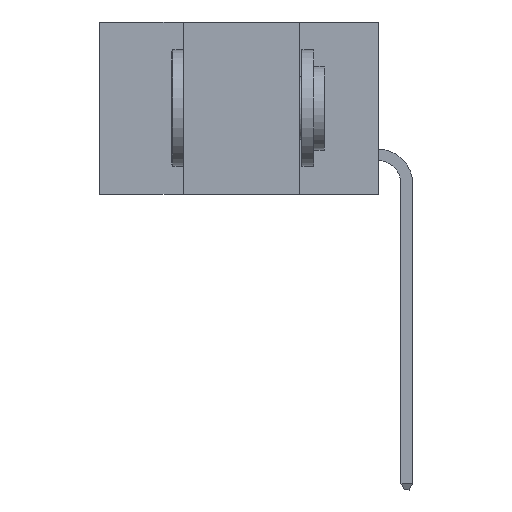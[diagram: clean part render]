
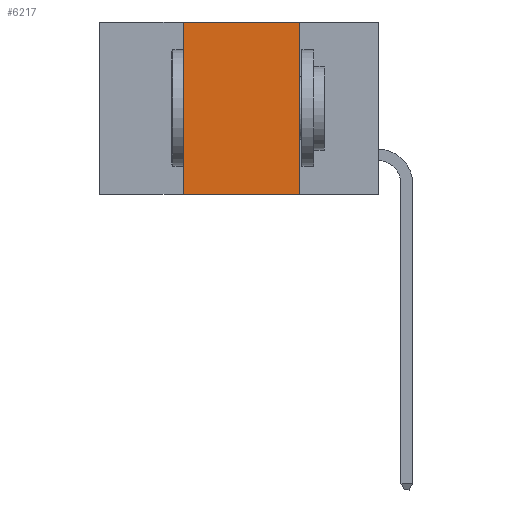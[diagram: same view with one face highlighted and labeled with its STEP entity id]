
A CAD part, left-side view. The second image highlights one B-rep face of the part: STEP entity #6217.
In plain terms, the highlighted planar face has unit normal (-1, 0, 0).
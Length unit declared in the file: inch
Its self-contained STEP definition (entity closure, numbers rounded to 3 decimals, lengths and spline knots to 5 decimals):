
#37 = CARTESIAN_POINT ( 'NONE',  ( 0., 0.42, -0.37 ) ) ;
#52 = EDGE_CURVE ( 'NONE', #8382, #4090, #4246, .T. ) ;
#571 = CARTESIAN_POINT ( 'NONE',  ( 0., 0.42, 0. ) ) ;
#820 = LINE ( 'NONE', #7157, #6916 ) ;
#878 = VERTEX_POINT ( 'NONE', #37 ) ;
#920 = CARTESIAN_POINT ( 'NONE',  ( 0., 0.17, 0. ) ) ;
#1599 = DIRECTION ( 'NONE',  ( 0., -1., 0. ) ) ;
#2435 = DIRECTION ( 'NONE',  ( 1., 0., 0. ) ) ;
#2514 = ORIENTED_EDGE ( 'NONE', *, *, #12529, .F. ) ;
#2537 = FACE_OUTER_BOUND ( 'NONE', #6471, .T. ) ;
#2568 = PLANE ( 'NONE',  #7795 ) ;
#2793 = ORIENTED_EDGE ( 'NONE', *, *, #52, .F. ) ;
#2965 = EDGE_CURVE ( 'NONE', #878, #4177, #820, .T. ) ;
#4090 = VERTEX_POINT ( 'NONE', #9179 ) ;
#4177 = VERTEX_POINT ( 'NONE', #9728 ) ;
#4246 = LINE ( 'NONE', #11647, #11690 ) ;
#5593 = ORIENTED_EDGE ( 'NONE', *, *, #2965, .T. ) ;
#6217 = ADVANCED_FACE ( 'NONE', ( #2537 ), #2568, .F. ) ;
#6471 = EDGE_LOOP ( 'NONE', ( #10758, #2793, #2514, #5593 ) ) ;
#6916 = VECTOR ( 'NONE', #7297, 39.37008 ) ;
#6940 = LINE ( 'NONE', #11303, #9209 ) ;
#7157 = CARTESIAN_POINT ( 'NONE',  ( 0., 0.6, -0.37 ) ) ;
#7297 = DIRECTION ( 'NONE',  ( 0., -1., 0. ) ) ;
#7506 = DIRECTION ( 'NONE',  ( 0., 0., -1. ) ) ;
#7795 = AXIS2_PLACEMENT_3D ( 'NONE', #8450, #2435, #7506 ) ;
#8175 = VECTOR ( 'NONE', #10060, 39.37008 ) ;
#8382 = VERTEX_POINT ( 'NONE', #571 ) ;
#8450 = CARTESIAN_POINT ( 'NONE',  ( 0., 0.6, 0. ) ) ;
#8650 = EDGE_CURVE ( 'NONE', #4090, #4177, #10730, .T. ) ;
#9179 = CARTESIAN_POINT ( 'NONE',  ( 0., 0.17, 0. ) ) ;
#9209 = VECTOR ( 'NONE', #12388, 39.37008 ) ;
#9728 = CARTESIAN_POINT ( 'NONE',  ( 0., 0.17, -0.37 ) ) ;
#10060 = DIRECTION ( 'NONE',  ( 0., 0., -1. ) ) ;
#10730 = LINE ( 'NONE', #920, #8175 ) ;
#10758 = ORIENTED_EDGE ( 'NONE', *, *, #8650, .F. ) ;
#11303 = CARTESIAN_POINT ( 'NONE',  ( 0., 0.42, 0. ) ) ;
#11647 = CARTESIAN_POINT ( 'NONE',  ( 0., 0.6, 0. ) ) ;
#11690 = VECTOR ( 'NONE', #1599, 39.37008 ) ;
#12388 = DIRECTION ( 'NONE',  ( 0., 0., 1. ) ) ;
#12529 = EDGE_CURVE ( 'NONE', #878, #8382, #6940, .T. ) ;
